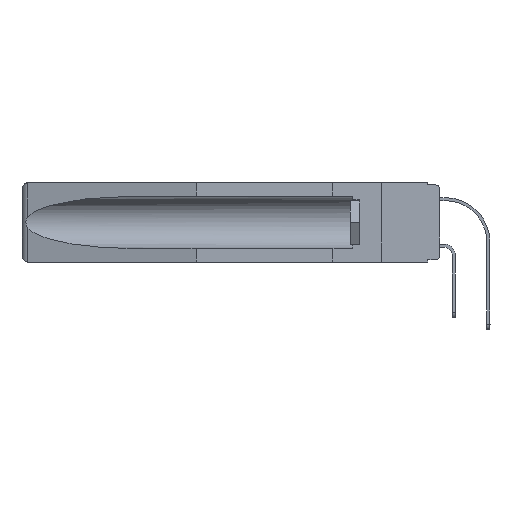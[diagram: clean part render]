
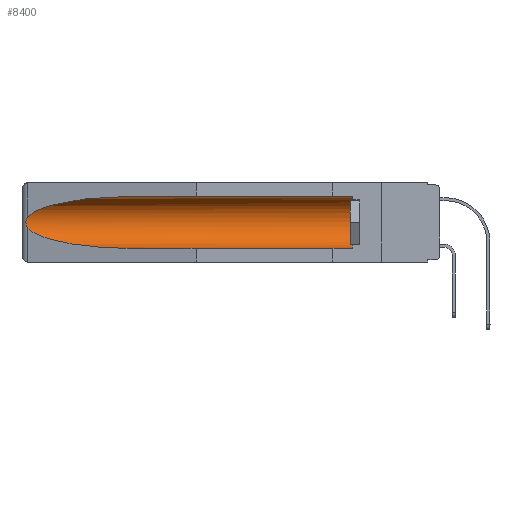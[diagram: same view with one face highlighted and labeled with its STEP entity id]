
A CAD part, left-side view. The second image highlights one B-rep face of the part: STEP entity #8400.
In plain terms, the highlighted cylindrical face has radius 2.857 mm (diameter 5.715 mm), a partial arc.
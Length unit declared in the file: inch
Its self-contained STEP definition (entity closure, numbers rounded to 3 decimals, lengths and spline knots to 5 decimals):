
#2014 = VERTEX_POINT ( 'NONE', #5545 ) ;
#2221 = CARTESIAN_POINT ( 'NONE',  ( 0.155, -0.30754, -0.1715 ) ) ;
#2530 = CARTESIAN_POINT ( 'NONE',  ( 0.2675, 1.53308, -0.16763 ) ) ;
#3352 = CARTESIAN_POINT ( 'NONE',  ( 0.26537, 1.52718, -0.19328 ) ) ;
#4778 = CARTESIAN_POINT ( 'NONE',  ( 0.21114, 1.30732, -0.284 ) ) ;
#4896 = CARTESIAN_POINT ( 'NONE',  ( 0.26597, 1.52961, -0.15275 ) ) ;
#5414 = CARTESIAN_POINT ( 'NONE',  ( 0.26537, 1.52718, -0.19328 ) ) ;
#5545 = CARTESIAN_POINT ( 'NONE',  ( 0.155, 0.126, -0.284 ) ) ;
#6235 = CARTESIAN_POINT ( 'NONE',  ( 0.155, 0.126, -0.1715 ) ) ;
#6257 = DIRECTION ( 'NONE',  ( 0., 1., 0. ) ) ;
#6261 =( BOUNDED_CURVE ( )  B_SPLINE_CURVE ( 3, ( #3352, #20328, #4778, #7389 ),
 .UNSPECIFIED., .F., .F. ) 
 B_SPLINE_CURVE_WITH_KNOTS ( ( 4, 4 ),
 ( 0.1948, 1.5708 ),
 .UNSPECIFIED. ) 
 CURVE ( )  GEOMETRIC_REPRESENTATION_ITEM ( )  RATIONAL_B_SPLINE_CURVE ( ( 1., 0.848, 0.848, 1. ) ) 
 REPRESENTATION_ITEM ( '' )  );
#6841 = CARTESIAN_POINT ( 'NONE',  ( 0.2675, 1.53308, -0.17534 ) ) ;
#6917 = CARTESIAN_POINT ( 'NONE',  ( 0.26537, 1.52718, -0.14972 ) ) ;
#7389 = CARTESIAN_POINT ( 'NONE',  ( 0.155, 1.07973, -0.284 ) ) ;
#8217 = CARTESIAN_POINT ( 'NONE',  ( 0.21114, 1.30732, -0.059 ) ) ;
#8312 = DIRECTION ( 'NONE',  ( 0., 0., 1. ) ) ;
#8400 = ADVANCED_FACE ( 'NONE', ( #20731 ), #14463, .F. ) ;
#8664 = CARTESIAN_POINT ( 'NONE',  ( 0.155, 0.126, -0.059 ) ) ;
#10107 = DIRECTION ( 'NONE',  ( 0., 1., 0. ) ) ;
#10154 = CARTESIAN_POINT ( 'NONE',  ( 0.155, -0.30754, -0.284 ) ) ;
#10901 = ORIENTED_EDGE ( 'NONE', *, *, #15731, .T. ) ;
#11375 = CARTESIAN_POINT ( 'NONE',  ( 0.155, 1.07973, -0.059 ) ) ;
#11376 = VERTEX_POINT ( 'NONE', #8664 ) ;
#11893 = AXIS2_PLACEMENT_3D ( 'NONE', #2221, #6257, #12775 ) ;
#11961 = VECTOR ( 'NONE', #10107, 39.37008 ) ;
#12437 = VERTEX_POINT ( 'NONE', #11375 ) ;
#12775 = DIRECTION ( 'NONE',  ( 0., 0., 1. ) ) ;
#12820 = CARTESIAN_POINT ( 'NONE',  ( 0.2673, 1.5327, -0.16383 ) ) ;
#12959 = CARTESIAN_POINT ( 'NONE',  ( 0.26597, 1.5296, -0.19026 ) ) ;
#13102 = CARTESIAN_POINT ( 'NONE',  ( 0.26537, 1.52718, -0.19328 ) ) ;
#13235 = CARTESIAN_POINT ( 'NONE',  ( 0.2673, 1.53269, -0.17917 ) ) ;
#14433 = CARTESIAN_POINT ( 'NONE',  ( 0.155, -0.30754, -0.059 ) ) ;
#14463 = CYLINDRICAL_SURFACE ( 'NONE', #11893, 0.1125 ) ;
#14732 = ORIENTED_EDGE ( 'NONE', *, *, #19960, .T. ) ;
#15230 = VERTEX_POINT ( 'NONE', #17016 ) ;
#15731 = EDGE_CURVE ( 'NONE', #12437, #20655, #25433, .T. ) ;
#16264 = CIRCLE ( 'NONE', #19358, 0.1125 ) ;
#16441 = EDGE_LOOP ( 'NONE', ( #10901, #24972, #14732, #20925, #21717, #18695 ) ) ;
#17016 = CARTESIAN_POINT ( 'NONE',  ( 0.155, 1.07973, -0.284 ) ) ;
#17131 = VERTEX_POINT ( 'NONE', #5414 ) ;
#17369 = CARTESIAN_POINT ( 'NONE',  ( 0.25451, 1.48313, -0.09465 ) ) ;
#17573 = CARTESIAN_POINT ( 'NONE',  ( 0.26655, 1.53094, -0.18657 ) ) ;
#17648 = B_SPLINE_CURVE_WITH_KNOTS ( 'NONE', 3,
 ( #19103, #4896, #25487, #12820, #2530, #6841, #13235, #17573, #12959, #13102 ),
 .UNSPECIFIED., .F., .F.,
 ( 4, 2, 2, 2, 4 ),
 ( 0., 0.00029, 0.00058, 0.00087, 0.00117 ),
 .UNSPECIFIED. ) ;
#18655 = LINE ( 'NONE', #10154, #20140 ) ;
#18695 = ORIENTED_EDGE ( 'NONE', *, *, #23027, .T. ) ;
#19103 = CARTESIAN_POINT ( 'NONE',  ( 0.26537, 1.52718, -0.14972 ) ) ;
#19310 = CARTESIAN_POINT ( 'NONE',  ( 0.26537, 1.52718, -0.14972 ) ) ;
#19358 = AXIS2_PLACEMENT_3D ( 'NONE', #6235, #24881, #8312 ) ;
#19960 = EDGE_CURVE ( 'NONE', #17131, #15230, #6261, .T. ) ;
#20140 = VECTOR ( 'NONE', #22284, 39.37008 ) ;
#20328 = CARTESIAN_POINT ( 'NONE',  ( 0.25451, 1.48313, -0.24835 ) ) ;
#20554 = EDGE_CURVE ( 'NONE', #2014, #11376, #16264, .T. ) ;
#20655 = VERTEX_POINT ( 'NONE', #19310 ) ;
#20731 = FACE_OUTER_BOUND ( 'NONE', #16441, .T. ) ;
#20925 = ORIENTED_EDGE ( 'NONE', *, *, #27391, .F. ) ;
#21717 = ORIENTED_EDGE ( 'NONE', *, *, #20554, .T. ) ;
#22284 = DIRECTION ( 'NONE',  ( 0., 1., 0. ) ) ;
#23027 = EDGE_CURVE ( 'NONE', #11376, #12437, #23196, .T. ) ;
#23196 = LINE ( 'NONE', #14433, #11961 ) ;
#24881 = DIRECTION ( 'NONE',  ( 0., -1., 0. ) ) ;
#24972 = ORIENTED_EDGE ( 'NONE', *, *, #25417, .T. ) ;
#25323 = CARTESIAN_POINT ( 'NONE',  ( 0.155, 1.07973, -0.059 ) ) ;
#25417 = EDGE_CURVE ( 'NONE', #20655, #17131, #17648, .T. ) ;
#25433 =( BOUNDED_CURVE ( )  B_SPLINE_CURVE ( 3, ( #25323, #8217, #17369, #6917 ),
 .UNSPECIFIED., .F., .F. ) 
 B_SPLINE_CURVE_WITH_KNOTS ( ( 4, 4 ),
 ( 4.71239, 6.08839 ),
 .UNSPECIFIED. ) 
 CURVE ( )  GEOMETRIC_REPRESENTATION_ITEM ( )  RATIONAL_B_SPLINE_CURVE ( ( 1., 0.848, 0.848, 1. ) ) 
 REPRESENTATION_ITEM ( '' )  );
#25487 = CARTESIAN_POINT ( 'NONE',  ( 0.26654, 1.53092, -0.15636 ) ) ;
#27391 = EDGE_CURVE ( 'NONE', #2014, #15230, #18655, .T. ) ;
